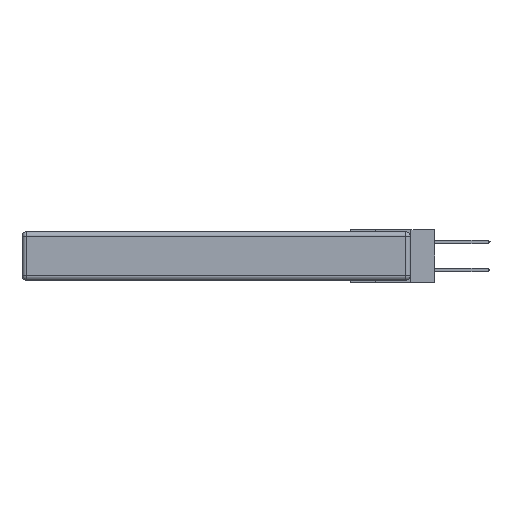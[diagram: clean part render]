
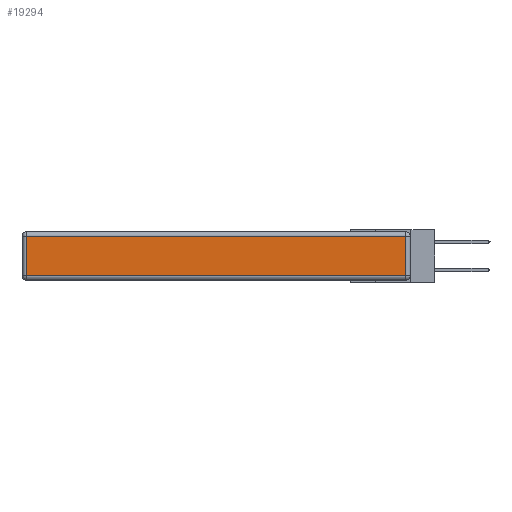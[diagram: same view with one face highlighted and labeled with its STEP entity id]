
A CAD part, left-side view. The second image highlights one B-rep face of the part: STEP entity #19294.
In plain terms, the highlighted planar face has unit normal (-1, 0, 0).
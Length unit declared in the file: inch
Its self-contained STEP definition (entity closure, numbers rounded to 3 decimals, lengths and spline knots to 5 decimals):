
#404 = EDGE_CURVE ( 'NONE', #24776, #11632, #11520, .T. ) ;
#1562 = CARTESIAN_POINT ( 'NONE',  ( 0., 2.72, -0.03 ) ) ;
#3332 = LINE ( 'NONE', #21730, #23287 ) ;
#3523 = CARTESIAN_POINT ( 'NONE',  ( 0., 2.75, -0.03 ) ) ;
#3808 = ORIENTED_EDGE ( 'NONE', *, *, #404, .T. ) ;
#4572 = EDGE_CURVE ( 'NONE', #5101, #19726, #18558, .T. ) ;
#4588 = VECTOR ( 'NONE', #13810, 39.37008 ) ;
#5101 = VERTEX_POINT ( 'NONE', #22917 ) ;
#5256 = ORIENTED_EDGE ( 'NONE', *, *, #4572, .T. ) ;
#5614 = PLANE ( 'NONE',  #20510 ) ;
#5980 = CARTESIAN_POINT ( 'NONE',  ( 0., 0., -0.343 ) ) ;
#7273 = FACE_OUTER_BOUND ( 'NONE', #18349, .T. ) ;
#7349 = CARTESIAN_POINT ( 'NONE',  ( 0., 0., -0.313 ) ) ;
#7476 = CARTESIAN_POINT ( 'NONE',  ( 0., 0.03, -0.313 ) ) ;
#8225 = ORIENTED_EDGE ( 'NONE', *, *, #15908, .T. ) ;
#8233 = EDGE_CURVE ( 'NONE', #19726, #24776, #15846, .T. ) ;
#11520 = LINE ( 'NONE', #7349, #17162 ) ;
#11632 = VERTEX_POINT ( 'NONE', #7476 ) ;
#13610 = DIRECTION ( 'NONE',  ( 0., 1., 0. ) ) ;
#13810 = DIRECTION ( 'NONE',  ( 0., 0., -1. ) ) ;
#14744 = CARTESIAN_POINT ( 'NONE',  ( 0., 2.72, -0.313 ) ) ;
#15604 = DIRECTION ( 'NONE',  ( -1., 0., 0. ) ) ;
#15846 = LINE ( 'NONE', #15915, #4588 ) ;
#15908 = EDGE_CURVE ( 'NONE', #11632, #5101, #3332, .T. ) ;
#15915 = CARTESIAN_POINT ( 'NONE',  ( 0., 2.72, -0.343 ) ) ;
#17162 = VECTOR ( 'NONE', #25347, 39.37008 ) ;
#18349 = EDGE_LOOP ( 'NONE', ( #3808, #8225, #5256, #22451 ) ) ;
#18558 = LINE ( 'NONE', #3523, #23219 ) ;
#19294 = ADVANCED_FACE ( 'NONE', ( #7273 ), #5614, .T. ) ;
#19726 = VERTEX_POINT ( 'NONE', #1562 ) ;
#20510 = AXIS2_PLACEMENT_3D ( 'NONE', #5980, #15604, #21694 ) ;
#21694 = DIRECTION ( 'NONE',  ( 0., 0., 1. ) ) ;
#21730 = CARTESIAN_POINT ( 'NONE',  ( 0., 0.03, -0.343 ) ) ;
#22451 = ORIENTED_EDGE ( 'NONE', *, *, #8233, .T. ) ;
#22917 = CARTESIAN_POINT ( 'NONE',  ( 0., 0.03, -0.03 ) ) ;
#23219 = VECTOR ( 'NONE', #13610, 39.37008 ) ;
#23287 = VECTOR ( 'NONE', #25740, 39.37008 ) ;
#24776 = VERTEX_POINT ( 'NONE', #14744 ) ;
#25347 = DIRECTION ( 'NONE',  ( 0., -1., 0. ) ) ;
#25740 = DIRECTION ( 'NONE',  ( 0., 0., 1. ) ) ;
